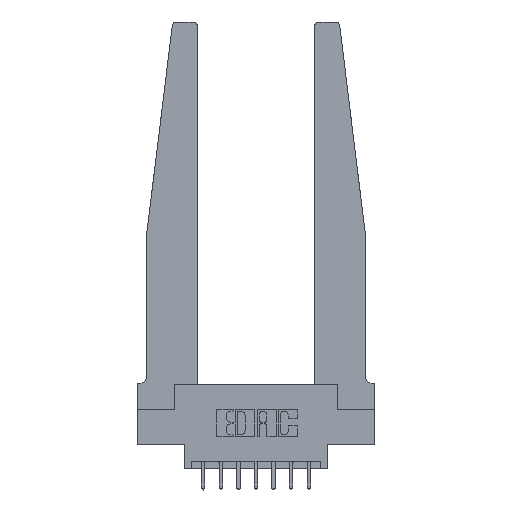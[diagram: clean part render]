
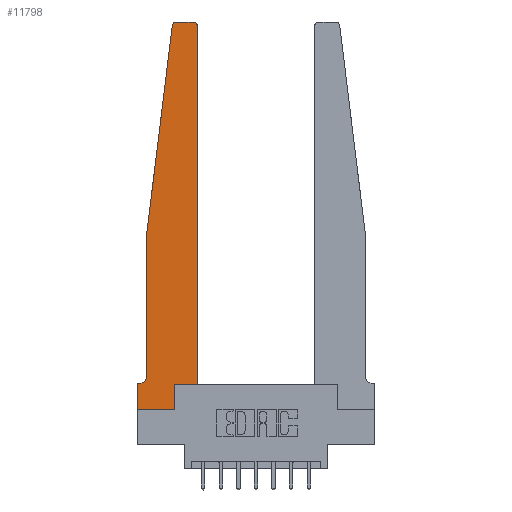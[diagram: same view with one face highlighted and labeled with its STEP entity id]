
A CAD part, top view. The second image highlights one B-rep face of the part: STEP entity #11798.
In plain terms, the highlighted planar face has unit normal (0, 0, 1).
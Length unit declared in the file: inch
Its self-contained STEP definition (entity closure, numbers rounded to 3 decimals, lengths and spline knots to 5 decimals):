
#106 = VECTOR ( 'NONE', #8998, 39.37008 ) ;
#390 = DIRECTION ( 'NONE',  ( -1., 0., 0. ) ) ;
#511 = AXIS2_PLACEMENT_3D ( 'NONE', #6594, #10517, #5023 ) ;
#538 = ORIENTED_EDGE ( 'NONE', *, *, #3822, .T. ) ;
#699 = EDGE_CURVE ( 'NONE', #1632, #5475, #7290, .T. ) ;
#798 = CARTESIAN_POINT ( 'NONE',  ( 0.395, 2.75, 0.37 ) ) ;
#888 = EDGE_CURVE ( 'NONE', #3184, #6372, #10967, .T. ) ;
#973 = ORIENTED_EDGE ( 'NONE', *, *, #3300, .T. ) ;
#1147 = CARTESIAN_POINT ( 'NONE',  ( 0.395, 2.72, 0.37 ) ) ;
#1154 = CARTESIAN_POINT ( 'NONE',  ( 0.425, 0.18, 0.37 ) ) ;
#1313 = DIRECTION ( 'NONE',  ( 0., 1., 0. ) ) ;
#1567 = EDGE_CURVE ( 'NONE', #12191, #2782, #8802, .T. ) ;
#1582 = CARTESIAN_POINT ( 'NONE',  ( 0.2605, 0.18, 0.37 ) ) ;
#1586 = ORIENTED_EDGE ( 'NONE', *, *, #12007, .T. ) ;
#1632 = VERTEX_POINT ( 'NONE', #2504 ) ;
#2236 = VERTEX_POINT ( 'NONE', #8674 ) ;
#2375 = DIRECTION ( 'NONE',  ( 1., 0., 0. ) ) ;
#2502 = LINE ( 'NONE', #1154, #106 ) ;
#2504 = CARTESIAN_POINT ( 'NONE',  ( 0.015, 0.1875, 0.37 ) ) ;
#2542 = ORIENTED_EDGE ( 'NONE', *, *, #10193, .T. ) ;
#2782 = VERTEX_POINT ( 'NONE', #12364 ) ;
#2911 = AXIS2_PLACEMENT_3D ( 'NONE', #13542, #7183, #390 ) ;
#3184 = VERTEX_POINT ( 'NONE', #9117 ) ;
#3200 = CARTESIAN_POINT ( 'NONE',  ( 0.425, 2.72, 0.37 ) ) ;
#3204 = VERTEX_POINT ( 'NONE', #9066 ) ;
#3300 = EDGE_CURVE ( 'NONE', #9635, #3204, #14040, .T. ) ;
#3412 = EDGE_CURVE ( 'NONE', #4675, #3184, #4149, .T. ) ;
#3413 = DIRECTION ( 'NONE',  ( -1., 0., 0. ) ) ;
#3822 = EDGE_CURVE ( 'NONE', #5475, #9635, #13704, .T. ) ;
#3876 = CIRCLE ( 'NONE', #5738, 0.03 ) ;
#3927 = CARTESIAN_POINT ( 'NONE',  ( 0.065, 1.25, 0.37 ) ) ;
#3979 = CARTESIAN_POINT ( 'NONE',  ( 0., 0., 0.37 ) ) ;
#4070 = DIRECTION ( 'NONE',  ( 0., -1., 0. ) ) ;
#4149 = LINE ( 'NONE', #7513, #12091 ) ;
#4225 = ORIENTED_EDGE ( 'NONE', *, *, #8425, .T. ) ;
#4323 = VECTOR ( 'NONE', #8420, 39.37008 ) ;
#4416 = ORIENTED_EDGE ( 'NONE', *, *, #7025, .T. ) ;
#4466 = VERTEX_POINT ( 'NONE', #3927 ) ;
#4675 = VERTEX_POINT ( 'NONE', #798 ) ;
#4777 = CARTESIAN_POINT ( 'NONE',  ( 0.425, 0.18, 0.37 ) ) ;
#4864 = ORIENTED_EDGE ( 'NONE', *, *, #699, .T. ) ;
#5023 = DIRECTION ( 'NONE',  ( 1., 0., 0. ) ) ;
#5054 = EDGE_CURVE ( 'NONE', #2236, #1632, #9567, .T. ) ;
#5139 = PLANE ( 'NONE',  #13197 ) ;
#5351 = FACE_OUTER_BOUND ( 'NONE', #11201, .T. ) ;
#5475 = VERTEX_POINT ( 'NONE', #7828 ) ;
#5738 = AXIS2_PLACEMENT_3D ( 'NONE', #1147, #8996, #2375 ) ;
#5911 = VECTOR ( 'NONE', #10414, 39.37008 ) ;
#6372 = VERTEX_POINT ( 'NONE', #9325 ) ;
#6594 = CARTESIAN_POINT ( 'NONE',  ( 0.27653, 2.72, 0.37 ) ) ;
#7025 = EDGE_CURVE ( 'NONE', #10289, #4675, #3876, .T. ) ;
#7183 = DIRECTION ( 'NONE',  ( 0., 0., -1. ) ) ;
#7245 = LINE ( 'NONE', #7337, #4323 ) ;
#7290 = LINE ( 'NONE', #12155, #9815 ) ;
#7337 = CARTESIAN_POINT ( 'NONE',  ( 0.065, 1.25, 0.37 ) ) ;
#7339 = DIRECTION ( 'NONE',  ( 1., 0., 0. ) ) ;
#7398 = ORIENTED_EDGE ( 'NONE', *, *, #888, .T. ) ;
#7513 = CARTESIAN_POINT ( 'NONE',  ( 0.25, 2.75, 0.37 ) ) ;
#7615 = DIRECTION ( 'NONE',  ( -1., 0., 0. ) ) ;
#7828 = CARTESIAN_POINT ( 'NONE',  ( 0., 0.1875, 0.37 ) ) ;
#7918 = DIRECTION ( 'NONE',  ( -0.122, -0.992, 0. ) ) ;
#8063 = CARTESIAN_POINT ( 'NONE',  ( 0.2605, 0.18, 0.37 ) ) ;
#8074 = VECTOR ( 'NONE', #4070, 39.37008 ) ;
#8294 = CARTESIAN_POINT ( 'NONE',  ( 0., 0., 0.37 ) ) ;
#8420 = DIRECTION ( 'NONE',  ( 0., -1., 0. ) ) ;
#8425 = EDGE_CURVE ( 'NONE', #6372, #4466, #11652, .T. ) ;
#8431 = DIRECTION ( 'NONE',  ( 1., 0., 0. ) ) ;
#8674 = CARTESIAN_POINT ( 'NONE',  ( 0.065, 0.2375, 0.37 ) ) ;
#8802 = LINE ( 'NONE', #4777, #5911 ) ;
#8996 = DIRECTION ( 'NONE',  ( 0., 0., 1. ) ) ;
#8998 = DIRECTION ( 'NONE',  ( 0., 1., 0. ) ) ;
#9066 = CARTESIAN_POINT ( 'NONE',  ( 0.2605, 0., 0.37 ) ) ;
#9117 = CARTESIAN_POINT ( 'NONE',  ( 0.27653, 2.75, 0.37 ) ) ;
#9222 = ORIENTED_EDGE ( 'NONE', *, *, #13734, .T. ) ;
#9325 = CARTESIAN_POINT ( 'NONE',  ( 0.24675, 2.72367, 0.37 ) ) ;
#9567 = CIRCLE ( 'NONE', #2911, 0.05 ) ;
#9635 = VERTEX_POINT ( 'NONE', #12620 ) ;
#9815 = VECTOR ( 'NONE', #3413, 39.37008 ) ;
#9963 = ORIENTED_EDGE ( 'NONE', *, *, #1567, .T. ) ;
#10193 = EDGE_CURVE ( 'NONE', #4466, #2236, #7245, .T. ) ;
#10289 = VERTEX_POINT ( 'NONE', #3200 ) ;
#10414 = DIRECTION ( 'NONE',  ( 1., 0., 0. ) ) ;
#10517 = DIRECTION ( 'NONE',  ( 0., 0., 1. ) ) ;
#10651 = VECTOR ( 'NONE', #7918, 39.37008 ) ;
#10934 = VECTOR ( 'NONE', #8431, 39.37008 ) ;
#10967 = CIRCLE ( 'NONE', #511, 0.03 ) ;
#11201 = EDGE_LOOP ( 'NONE', ( #11829, #7398, #4225, #2542, #12616, #4864, #538, #973, #9222, #9963, #1586, #4416 ) ) ;
#11652 = LINE ( 'NONE', #12158, #10651 ) ;
#11798 = ADVANCED_FACE ( 'NONE', ( #5351 ), #5139, .T. ) ;
#11829 = ORIENTED_EDGE ( 'NONE', *, *, #3412, .T. ) ;
#12007 = EDGE_CURVE ( 'NONE', #2782, #10289, #2502, .T. ) ;
#12091 = VECTOR ( 'NONE', #7615, 39.37008 ) ;
#12155 = CARTESIAN_POINT ( 'NONE',  ( 0.065, 0.1875, 0.37 ) ) ;
#12158 = CARTESIAN_POINT ( 'NONE',  ( 0.065, 1.25, 0.37 ) ) ;
#12191 = VERTEX_POINT ( 'NONE', #1582 ) ;
#12364 = CARTESIAN_POINT ( 'NONE',  ( 0.425, 0.18, 0.37 ) ) ;
#12599 = VECTOR ( 'NONE', #1313, 39.37008 ) ;
#12616 = ORIENTED_EDGE ( 'NONE', *, *, #5054, .T. ) ;
#12620 = CARTESIAN_POINT ( 'NONE',  ( 0., 0., 0.37 ) ) ;
#12650 = CARTESIAN_POINT ( 'NONE',  ( 0., 0.1875, 0.37 ) ) ;
#12828 = LINE ( 'NONE', #8063, #12599 ) ;
#13197 = AXIS2_PLACEMENT_3D ( 'NONE', #12650, #13683, #7339 ) ;
#13542 = CARTESIAN_POINT ( 'NONE',  ( 0.015, 0.2375, 0.37 ) ) ;
#13683 = DIRECTION ( 'NONE',  ( 0., 0., 1. ) ) ;
#13704 = LINE ( 'NONE', #3979, #8074 ) ;
#13734 = EDGE_CURVE ( 'NONE', #3204, #12191, #12828, .T. ) ;
#14040 = LINE ( 'NONE', #8294, #10934 ) ;
